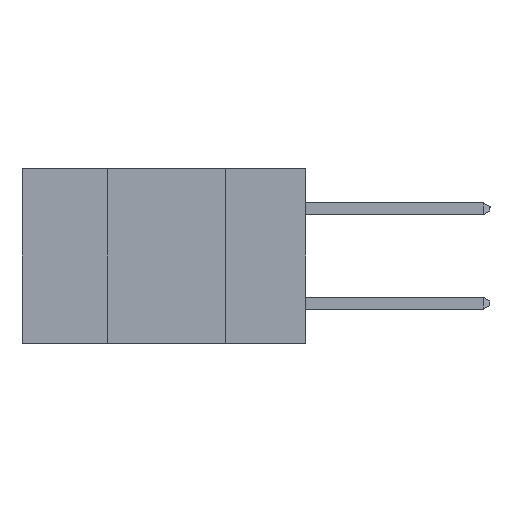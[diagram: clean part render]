
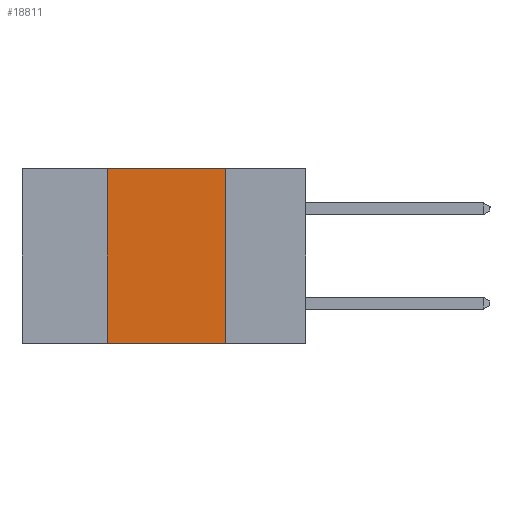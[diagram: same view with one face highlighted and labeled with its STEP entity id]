
A CAD part, left-side view. The second image highlights one B-rep face of the part: STEP entity #18811.
In plain terms, the highlighted planar face has unit normal (-1, 0, 0).
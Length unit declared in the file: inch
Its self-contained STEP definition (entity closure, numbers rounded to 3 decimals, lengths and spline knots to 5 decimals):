
#387 = EDGE_CURVE ( 'NONE', #11998, #23887, #5233, .T. ) ;
#411 = CARTESIAN_POINT ( 'NONE',  ( 0., 0.6, -0.37 ) ) ;
#470 = VERTEX_POINT ( 'NONE', #22033 ) ;
#2301 = VECTOR ( 'NONE', #10407, 39.37008 ) ;
#3078 = VECTOR ( 'NONE', #14085, 39.37008 ) ;
#5233 = LINE ( 'NONE', #13463, #13102 ) ;
#5384 = CARTESIAN_POINT ( 'NONE',  ( 0., 0.6, 0. ) ) ;
#5401 = EDGE_CURVE ( 'NONE', #12157, #11998, #11990, .T. ) ;
#5779 = ORIENTED_EDGE ( 'NONE', *, *, #6091, .F. ) ;
#6091 = EDGE_CURVE ( 'NONE', #470, #12157, #13003, .T. ) ;
#6204 = EDGE_LOOP ( 'NONE', ( #10507, #15760, #5779, #11349 ) ) ;
#9133 = FACE_OUTER_BOUND ( 'NONE', #6204, .T. ) ;
#9236 = DIRECTION ( 'NONE',  ( 0., 0., -1. ) ) ;
#10407 = DIRECTION ( 'NONE',  ( 0., -1., 0. ) ) ;
#10507 = ORIENTED_EDGE ( 'NONE', *, *, #387, .F. ) ;
#11122 = DIRECTION ( 'NONE',  ( 0., 0., -1. ) ) ;
#11349 = ORIENTED_EDGE ( 'NONE', *, *, #17760, .T. ) ;
#11990 = LINE ( 'NONE', #18064, #3078 ) ;
#11998 = VERTEX_POINT ( 'NONE', #18612 ) ;
#12157 = VERTEX_POINT ( 'NONE', #17535 ) ;
#13003 = LINE ( 'NONE', #21056, #20379 ) ;
#13102 = VECTOR ( 'NONE', #9236, 39.37008 ) ;
#13463 = CARTESIAN_POINT ( 'NONE',  ( 0., 0.17, -0.37 ) ) ;
#14085 = DIRECTION ( 'NONE',  ( 0., -1., 0. ) ) ;
#15760 = ORIENTED_EDGE ( 'NONE', *, *, #5401, .F. ) ;
#16711 = DIRECTION ( 'NONE',  ( 0., 0., 1. ) ) ;
#16767 = CARTESIAN_POINT ( 'NONE',  ( 0., 0.17, -0.37 ) ) ;
#17535 = CARTESIAN_POINT ( 'NONE',  ( 0., 0.42, 0. ) ) ;
#17760 = EDGE_CURVE ( 'NONE', #470, #23887, #20453, .T. ) ;
#18064 = CARTESIAN_POINT ( 'NONE',  ( 0., 0.6, 0. ) ) ;
#18612 = CARTESIAN_POINT ( 'NONE',  ( 0., 0.17, 0. ) ) ;
#18811 = ADVANCED_FACE ( 'NONE', ( #9133 ), #19318, .F. ) ;
#19318 = PLANE ( 'NONE',  #20134 ) ;
#20134 = AXIS2_PLACEMENT_3D ( 'NONE', #5384, #23532, #11122 ) ;
#20379 = VECTOR ( 'NONE', #16711, 39.37008 ) ;
#20453 = LINE ( 'NONE', #411, #2301 ) ;
#21056 = CARTESIAN_POINT ( 'NONE',  ( 0., 0.42, -0.37 ) ) ;
#22033 = CARTESIAN_POINT ( 'NONE',  ( 0., 0.42, -0.37 ) ) ;
#23532 = DIRECTION ( 'NONE',  ( 1., 0., 0. ) ) ;
#23887 = VERTEX_POINT ( 'NONE', #16767 ) ;
